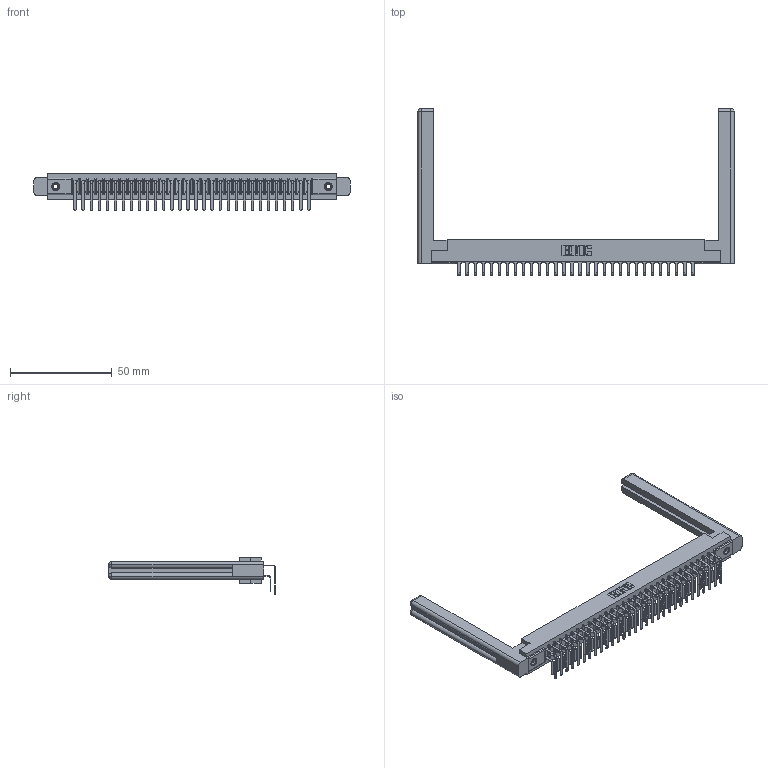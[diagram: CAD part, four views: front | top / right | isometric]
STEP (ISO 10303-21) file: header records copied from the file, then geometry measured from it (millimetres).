
FILE_DESCRIPTION (( 'STEP AP203' ), '1' );
FILE_NAME ('357-030-459-158.STEP', '2020-10-02T01:18:53', ( '' ), ( '' ), 'SwSTEP 2.0', 'SolidWorks 2020', '' );
FILE_SCHEMA (( 'CONFIG_CONTROL_DESIGN' ));
Length unit declared in the file: inch
Products named in the file (6): 307-220-058; 307-290-001_558 559 - 1 (Single); 357-030-459-158; 307 Part_.156 Dia Mounting Holes; 345-250-001_345-250-001-102; 307-290-001_559 - 2 (Single)
Assembly tree (65 placements, depth 2):
  357-030-459-158
    307 Part_.156 Dia Mounting Holes
    307-290-001_558 559 - 1 (Single)  x30
    307-290-001_559 - 2 (Single)  x30
    307-220-058  x2
    345-250-001_345-250-001-102  x2
Bounding box: 155.5 x 82 x 18.07 mm (x, y, z)
Volume: 23845.8 mm3; surface area: 26654.4 mm2
Topology: 65 solids, 65 shells, 3291 faces, 9197 edges, 5954 vertices
Faces by surface type: plane 2134, cylinder 1071, sphere 62, torus 12, cone 12
Entity records: 32238 total; most frequent: CARTESIAN_POINT 5299, ORIENTED_EDGE 5192, DIRECTION 5152, EDGE_CURVE 2596, VECTOR 1982, LINE 1982, VERTEX_POINT 1678, AXIS2_PLACEMENT_3D 1585
